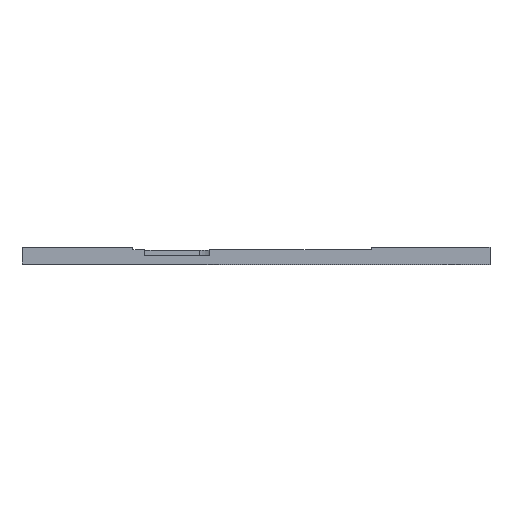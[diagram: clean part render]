
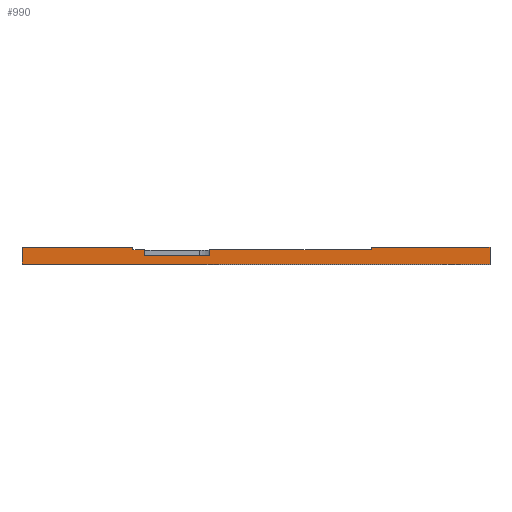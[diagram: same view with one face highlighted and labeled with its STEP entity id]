
A CAD part, top view. The second image highlights one B-rep face of the part: STEP entity #990.
In plain terms, the highlighted planar face has unit normal (0, 0, 1).
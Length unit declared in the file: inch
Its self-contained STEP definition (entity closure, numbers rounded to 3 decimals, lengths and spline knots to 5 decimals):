
#16 = CARTESIAN_POINT ( 'NONE',  ( 0.9135, -0.06, 0. ) ) ;
#31 = LINE ( 'NONE', #651, #849 ) ;
#33 = ORIENTED_EDGE ( 'NONE', *, *, #714, .T. ) ;
#99 = ORIENTED_EDGE ( 'NONE', *, *, #890, .F. ) ;
#100 = DIRECTION ( 'NONE',  ( 1., 0., 0. ) ) ;
#101 = DIRECTION ( 'NONE',  ( 0., 0., 1. ) ) ;
#105 = PLANE ( 'NONE',  #1099 ) ;
#128 = CARTESIAN_POINT ( 'NONE',  ( 0., -0.125, 0. ) ) ;
#147 = ORIENTED_EDGE ( 'NONE', *, *, #842, .F. ) ;
#154 = VECTOR ( 'NONE', #333, 39.37008 ) ;
#169 = CARTESIAN_POINT ( 'NONE',  ( 0., -0.06, 0. ) ) ;
#173 = DIRECTION ( 'NONE',  ( 1., 0., 0. ) ) ;
#175 = VERTEX_POINT ( 'NONE', #1129 ) ;
#184 = VECTOR ( 'NONE', #1005, 39.37008 ) ;
#203 = CARTESIAN_POINT ( 'NONE',  ( 0., -0.018, 0. ) ) ;
#204 = DIRECTION ( 'NONE',  ( 1., 0., 0. ) ) ;
#286 = CARTESIAN_POINT ( 'NONE',  ( 0.9135, -0.06, 0. ) ) ;
#287 = DIRECTION ( 'NONE',  ( 0., 1., 0. ) ) ;
#320 = DIRECTION ( 'NONE',  ( 1., 0., 0. ) ) ;
#322 = CARTESIAN_POINT ( 'NONE',  ( 0.827, -0.018, 0. ) ) ;
#331 = CARTESIAN_POINT ( 'NONE',  ( 0., -0.018, 0. ) ) ;
#333 = DIRECTION ( 'NONE',  ( 0., 1., 0. ) ) ;
#335 = LINE ( 'NONE', #554, #888 ) ;
#351 = VECTOR ( 'NONE', #354, 39.37008 ) ;
#352 = CARTESIAN_POINT ( 'NONE',  ( 1.3985, -0.06, 0. ) ) ;
#354 = DIRECTION ( 'NONE',  ( 0., 1., 0. ) ) ;
#387 = CARTESIAN_POINT ( 'NONE',  ( 0.827, -0.018, 0. ) ) ;
#398 = VERTEX_POINT ( 'NONE', #1014 ) ;
#414 = EDGE_CURVE ( 'NONE', #175, #488, #897, .T. ) ;
#424 = VECTOR ( 'NONE', #950, 39.37008 ) ;
#445 = VERTEX_POINT ( 'NONE', #1109 ) ;
#451 = FACE_OUTER_BOUND ( 'NONE', #477, .T. ) ;
#465 = VERTEX_POINT ( 'NONE', #1032 ) ;
#469 = LINE ( 'NONE', #286, #729 ) ;
#472 = ORIENTED_EDGE ( 'NONE', *, *, #547, .F. ) ;
#477 = EDGE_LOOP ( 'NONE', ( #147, #940, #726, #686, #99, #996, #979, #1100, #1190, #33, #472, #1135 ) ) ;
#488 = VERTEX_POINT ( 'NONE', #941 ) ;
#495 = DIRECTION ( 'NONE',  ( 0., 1., 0. ) ) ;
#498 = EDGE_CURVE ( 'NONE', #576, #175, #1042, .T. ) ;
#529 = LINE ( 'NONE', #803, #550 ) ;
#533 = LINE ( 'NONE', #203, #1009 ) ;
#545 = VERTEX_POINT ( 'NONE', #806 ) ;
#547 = EDGE_CURVE ( 'NONE', #465, #662, #529, .T. ) ;
#550 = VECTOR ( 'NONE', #807, 39.37008 ) ;
#554 = CARTESIAN_POINT ( 'NONE',  ( 3.49, -0.125, 0. ) ) ;
#557 = VERTEX_POINT ( 'NONE', #788 ) ;
#558 = CARTESIAN_POINT ( 'NONE',  ( 0., -0.125, 0. ) ) ;
#561 = DIRECTION ( 'NONE',  ( 1., 0., 0. ) ) ;
#576 = VERTEX_POINT ( 'NONE', #775 ) ;
#602 = VERTEX_POINT ( 'NONE', #755 ) ;
#628 = DIRECTION ( 'NONE',  ( 0., 1., 0. ) ) ;
#651 = CARTESIAN_POINT ( 'NONE',  ( 2.605, -0.018, 0. ) ) ;
#662 = VERTEX_POINT ( 'NONE', #672 ) ;
#666 = VECTOR ( 'NONE', #320, 39.37008 ) ;
#672 = CARTESIAN_POINT ( 'NONE',  ( 3.49, 0., 0. ) ) ;
#686 = ORIENTED_EDGE ( 'NONE', *, *, #858, .T. ) ;
#691 = EDGE_CURVE ( 'NONE', #545, #465, #31, .T. ) ;
#712 = EDGE_CURVE ( 'NONE', #576, #557, #866, .T. ) ;
#714 = EDGE_CURVE ( 'NONE', #557, #662, #335, .T. ) ;
#726 = ORIENTED_EDGE ( 'NONE', *, *, #904, .F. ) ;
#729 = VECTOR ( 'NONE', #287, 39.37008 ) ;
#755 = CARTESIAN_POINT ( 'NONE',  ( 1.3985, -0.018, 0. ) ) ;
#775 = CARTESIAN_POINT ( 'NONE',  ( 0., -0.125, 0. ) ) ;
#788 = CARTESIAN_POINT ( 'NONE',  ( 3.49, -0.125, 0. ) ) ;
#791 = VERTEX_POINT ( 'NONE', #387 ) ;
#803 = CARTESIAN_POINT ( 'NONE',  ( 0., 0., 0. ) ) ;
#806 = CARTESIAN_POINT ( 'NONE',  ( 2.605, -0.018, 0. ) ) ;
#807 = DIRECTION ( 'NONE',  ( 1., 0., 0. ) ) ;
#814 = EDGE_CURVE ( 'NONE', #398, #602, #1026, .T. ) ;
#842 = EDGE_CURVE ( 'NONE', #602, #545, #856, .T. ) ;
#846 = EDGE_CURVE ( 'NONE', #791, #488, #898, .T. ) ;
#849 = VECTOR ( 'NONE', #628, 39.37008 ) ;
#856 = LINE ( 'NONE', #331, #666 ) ;
#858 = EDGE_CURVE ( 'NONE', #1182, #445, #469, .T. ) ;
#859 = VECTOR ( 'NONE', #173, 39.37008 ) ;
#866 = LINE ( 'NONE', #558, #1044 ) ;
#888 = VECTOR ( 'NONE', #495, 39.37008 ) ;
#890 = EDGE_CURVE ( 'NONE', #791, #445, #533, .T. ) ;
#897 = LINE ( 'NONE', #1007, #184 ) ;
#898 = LINE ( 'NONE', #322, #154 ) ;
#904 = EDGE_CURVE ( 'NONE', #1182, #398, #1037, .T. ) ;
#923 = CARTESIAN_POINT ( 'NONE',  ( 0., -0.125, 0. ) ) ;
#940 = ORIENTED_EDGE ( 'NONE', *, *, #814, .F. ) ;
#941 = CARTESIAN_POINT ( 'NONE',  ( 0.827, 0., 0. ) ) ;
#950 = DIRECTION ( 'NONE',  ( 0., 1., 0. ) ) ;
#979 = ORIENTED_EDGE ( 'NONE', *, *, #414, .F. ) ;
#990 = ADVANCED_FACE ( 'NONE', ( #451 ), #105, .T. ) ;
#996 = ORIENTED_EDGE ( 'NONE', *, *, #846, .T. ) ;
#1005 = DIRECTION ( 'NONE',  ( 1., 0., 0. ) ) ;
#1007 = CARTESIAN_POINT ( 'NONE',  ( 0., 0., 0. ) ) ;
#1009 = VECTOR ( 'NONE', #204, 39.37008 ) ;
#1014 = CARTESIAN_POINT ( 'NONE',  ( 1.3985, -0.06, 0. ) ) ;
#1026 = LINE ( 'NONE', #352, #351 ) ;
#1032 = CARTESIAN_POINT ( 'NONE',  ( 2.605, 0., 0. ) ) ;
#1037 = LINE ( 'NONE', #169, #859 ) ;
#1042 = LINE ( 'NONE', #923, #424 ) ;
#1044 = VECTOR ( 'NONE', #561, 39.37008 ) ;
#1099 = AXIS2_PLACEMENT_3D ( 'NONE', #128, #101, #100 ) ;
#1100 = ORIENTED_EDGE ( 'NONE', *, *, #498, .F. ) ;
#1109 = CARTESIAN_POINT ( 'NONE',  ( 0.9135, -0.018, 0. ) ) ;
#1129 = CARTESIAN_POINT ( 'NONE',  ( 0., 0., 0. ) ) ;
#1135 = ORIENTED_EDGE ( 'NONE', *, *, #691, .F. ) ;
#1182 = VERTEX_POINT ( 'NONE', #16 ) ;
#1190 = ORIENTED_EDGE ( 'NONE', *, *, #712, .T. ) ;
